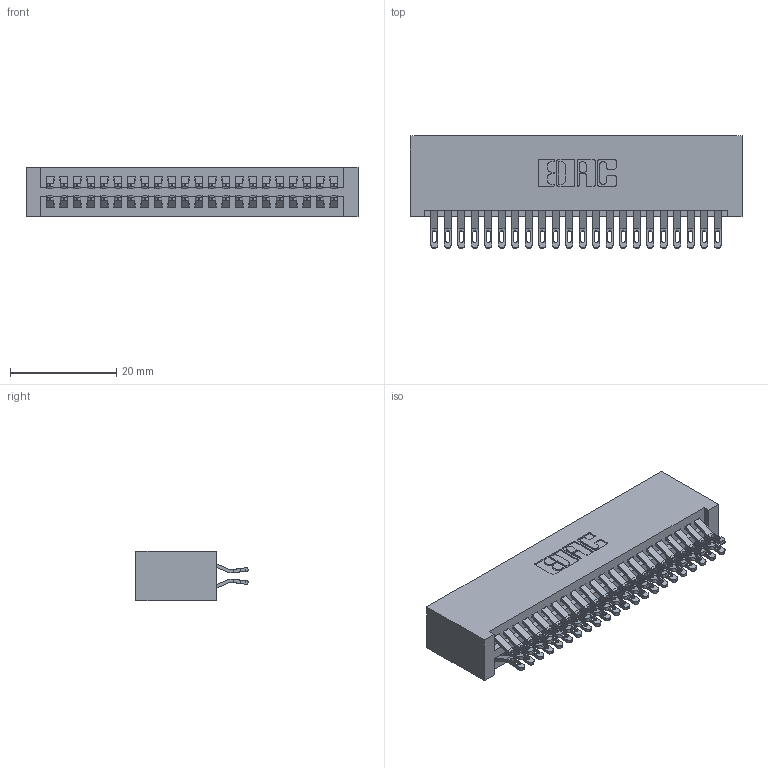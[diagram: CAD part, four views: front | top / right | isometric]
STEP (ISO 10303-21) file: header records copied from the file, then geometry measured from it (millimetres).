
FILE_DESCRIPTION (( 'STEP AP203' ), '1' );
FILE_NAME ('395-044-555-201.STEP', '2018-11-15T21:47:08', ( '' ), ( '' ), 'SwSTEP 2.0', 'SolidWorks 2016', '' );
FILE_SCHEMA (( 'CONFIG_CONTROL_DESIGN' ));
Length unit declared in the file: inch
Products named in the file (3): 345 Part_No Mounting Lugs; 395-044-555-201; 345-292-001_555 Tail
Assembly tree (45 placements, depth 2):
  395-044-555-201
    345 Part_No Mounting Lugs
    345-292-001_555 Tail  x44
Bounding box: 62.48 x 21.13 x 9.4 mm (x, y, z)
Volume: 6627.6 mm3; surface area: 10156.6 mm2
Topology: 45 solids, 45 shells, 2582 faces, 8105 edges, 5402 vertices
Faces by surface type: plane 1440, cylinder 1142
Entity records: 20003 total; most frequent: CARTESIAN_POINT 3406, ORIENTED_EDGE 3310, DIRECTION 2991, EDGE_CURVE 1655, VECTOR 1423, LINE 1423, VERTEX_POINT 1102, AXIS2_PLACEMENT_3D 784
